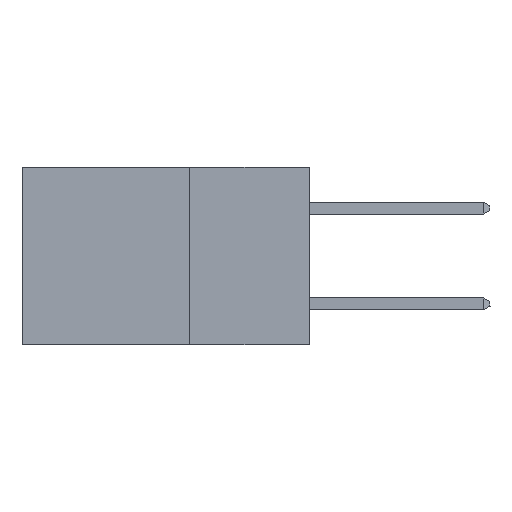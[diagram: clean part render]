
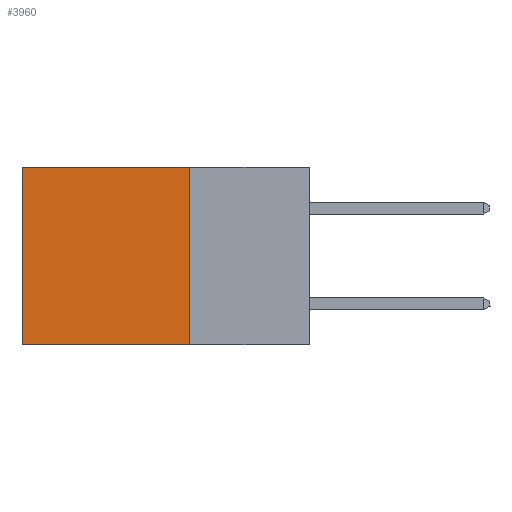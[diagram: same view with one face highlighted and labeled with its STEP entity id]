
A CAD part, left-side view. The second image highlights one B-rep face of the part: STEP entity #3960.
In plain terms, the highlighted planar face has unit normal (-1, 0, 0).
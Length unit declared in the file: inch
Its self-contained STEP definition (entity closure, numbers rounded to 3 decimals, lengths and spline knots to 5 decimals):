
#24 = AXIS2_PLACEMENT_3D ( 'NONE', #1026, #10551, #5116 ) ;
#228 = LINE ( 'NONE', #1632, #4069 ) ;
#509 = CARTESIAN_POINT ( 'NONE',  ( 0.2875, 0.6, 0. ) ) ;
#1026 = CARTESIAN_POINT ( 'NONE',  ( 0.2875, 0.25, 0. ) ) ;
#1293 = CARTESIAN_POINT ( 'NONE',  ( 0.2875, 0.25, 0. ) ) ;
#1495 = DIRECTION ( 'NONE',  ( 0., 0., -1. ) ) ;
#1510 = DIRECTION ( 'NONE',  ( 0., 1., 0. ) ) ;
#1632 = CARTESIAN_POINT ( 'NONE',  ( 0.2875, 0.25, -0.37 ) ) ;
#2185 = VERTEX_POINT ( 'NONE', #4051 ) ;
#2241 = EDGE_CURVE ( 'NONE', #9376, #4187, #228, .T. ) ;
#2307 = FACE_OUTER_BOUND ( 'NONE', #10893, .T. ) ;
#3232 = CARTESIAN_POINT ( 'NONE',  ( 0.2875, 0.25, 0. ) ) ;
#3788 = LINE ( 'NONE', #1293, #8467 ) ;
#3960 = ADVANCED_FACE ( 'NONE', ( #2307 ), #4140, .F. ) ;
#4051 = CARTESIAN_POINT ( 'NONE',  ( 0.2875, 0.6, 0. ) ) ;
#4069 = VECTOR ( 'NONE', #1510, 39.37008 ) ;
#4140 = PLANE ( 'NONE',  #24 ) ;
#4187 = VERTEX_POINT ( 'NONE', #7696 ) ;
#4318 = EDGE_CURVE ( 'NONE', #5894, #9376, #8006, .T. ) ;
#4814 = ORIENTED_EDGE ( 'NONE', *, *, #2241, .F. ) ;
#5116 = DIRECTION ( 'NONE',  ( 0., 0., -1. ) ) ;
#5611 = VECTOR ( 'NONE', #7091, 39.37008 ) ;
#5894 = VERTEX_POINT ( 'NONE', #12114 ) ;
#7091 = DIRECTION ( 'NONE',  ( 0., 0., -1. ) ) ;
#7231 = ORIENTED_EDGE ( 'NONE', *, *, #4318, .F. ) ;
#7696 = CARTESIAN_POINT ( 'NONE',  ( 0.2875, 0.6, -0.37 ) ) ;
#7870 = VECTOR ( 'NONE', #1495, 39.37008 ) ;
#8006 = LINE ( 'NONE', #3232, #5611 ) ;
#8467 = VECTOR ( 'NONE', #10807, 39.37008 ) ;
#9342 = EDGE_CURVE ( 'NONE', #5894, #2185, #3788, .T. ) ;
#9376 = VERTEX_POINT ( 'NONE', #11705 ) ;
#10394 = EDGE_CURVE ( 'NONE', #2185, #4187, #10834, .T. ) ;
#10551 = DIRECTION ( 'NONE',  ( 1., 0., 0. ) ) ;
#10807 = DIRECTION ( 'NONE',  ( 0., 1., 0. ) ) ;
#10834 = LINE ( 'NONE', #509, #7870 ) ;
#10893 = EDGE_LOOP ( 'NONE', ( #11693, #4814, #7231, #11962 ) ) ;
#11693 = ORIENTED_EDGE ( 'NONE', *, *, #10394, .T. ) ;
#11705 = CARTESIAN_POINT ( 'NONE',  ( 0.2875, 0.25, -0.37 ) ) ;
#11962 = ORIENTED_EDGE ( 'NONE', *, *, #9342, .T. ) ;
#12114 = CARTESIAN_POINT ( 'NONE',  ( 0.2875, 0.25, 0. ) ) ;
